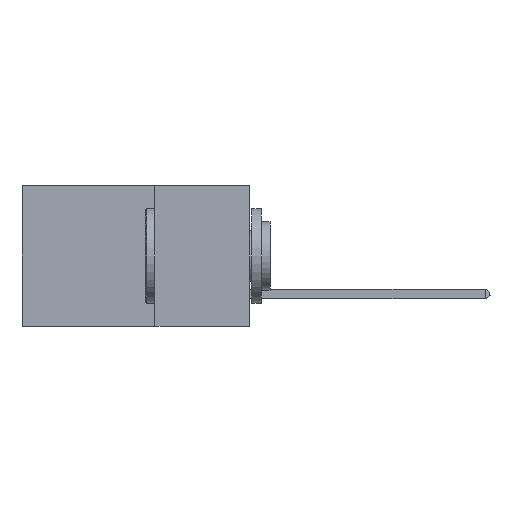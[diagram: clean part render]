
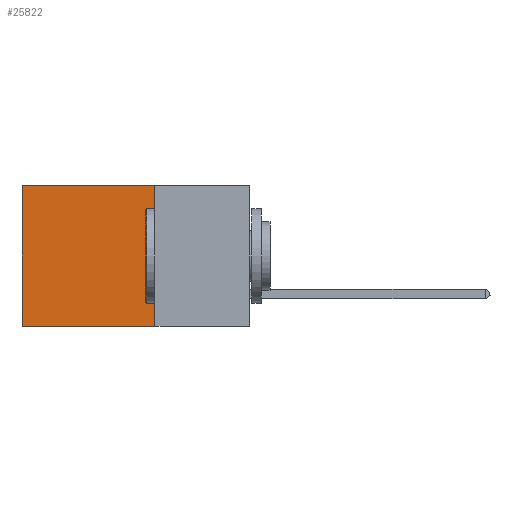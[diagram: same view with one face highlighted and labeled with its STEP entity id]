
A CAD part, left-side view. The second image highlights one B-rep face of the part: STEP entity #25822.
In plain terms, the highlighted planar face has unit normal (-1, 0, 0).
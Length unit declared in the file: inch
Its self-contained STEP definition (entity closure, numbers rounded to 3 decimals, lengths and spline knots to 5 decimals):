
#1035 = ORIENTED_EDGE ( 'NONE', *, *, #13545, .T. ) ;
#1721 = LINE ( 'NONE', #9431, #6981 ) ;
#2268 = ORIENTED_EDGE ( 'NONE', *, *, #10906, .T. ) ;
#4077 = DIRECTION ( 'NONE',  ( 0., 0., -1. ) ) ;
#4103 = VECTOR ( 'NONE', #25161, 39.37008 ) ;
#5337 = CARTESIAN_POINT ( 'NONE',  ( 0.2875, 0.6, 0. ) ) ;
#6981 = VECTOR ( 'NONE', #11683, 39.37008 ) ;
#7983 = VERTEX_POINT ( 'NONE', #5337 ) ;
#8752 = AXIS2_PLACEMENT_3D ( 'NONE', #27367, #15948, #20723 ) ;
#9068 = CARTESIAN_POINT ( 'NONE',  ( 0.2875, 0.25, 0. ) ) ;
#9376 = LINE ( 'NONE', #26934, #16824 ) ;
#9431 = CARTESIAN_POINT ( 'NONE',  ( 0.2875, 0.25, 0. ) ) ;
#10137 = LINE ( 'NONE', #22988, #4103 ) ;
#10906 = EDGE_CURVE ( 'NONE', #29170, #7983, #16612, .T. ) ;
#11400 = CARTESIAN_POINT ( 'NONE',  ( 0.2875, 0.25, -0.37 ) ) ;
#11448 = ORIENTED_EDGE ( 'NONE', *, *, #25806, .F. ) ;
#11585 = ORIENTED_EDGE ( 'NONE', *, *, #27945, .F. ) ;
#11683 = DIRECTION ( 'NONE',  ( 0., 0., -1. ) ) ;
#13518 = EDGE_LOOP ( 'NONE', ( #1035, #11585, #11448, #2268 ) ) ;
#13545 = EDGE_CURVE ( 'NONE', #7983, #23250, #9376, .T. ) ;
#13915 = CARTESIAN_POINT ( 'NONE',  ( 0.2875, 0.6, -0.37 ) ) ;
#15948 = DIRECTION ( 'NONE',  ( 1., 0., 0. ) ) ;
#16612 = LINE ( 'NONE', #9068, #28609 ) ;
#16824 = VECTOR ( 'NONE', #4077, 39.37008 ) ;
#20723 = DIRECTION ( 'NONE',  ( 0., 0., -1. ) ) ;
#21011 = VERTEX_POINT ( 'NONE', #11400 ) ;
#22988 = CARTESIAN_POINT ( 'NONE',  ( 0.2875, 0.25, -0.37 ) ) ;
#23250 = VERTEX_POINT ( 'NONE', #13915 ) ;
#24744 = CARTESIAN_POINT ( 'NONE',  ( 0.2875, 0.25, 0. ) ) ;
#25161 = DIRECTION ( 'NONE',  ( 0., 1., 0. ) ) ;
#25806 = EDGE_CURVE ( 'NONE', #29170, #21011, #1721, .T. ) ;
#25822 = ADVANCED_FACE ( 'NONE', ( #27819 ), #27461, .F. ) ;
#26934 = CARTESIAN_POINT ( 'NONE',  ( 0.2875, 0.6, 0. ) ) ;
#27101 = DIRECTION ( 'NONE',  ( 0., 1., 0. ) ) ;
#27367 = CARTESIAN_POINT ( 'NONE',  ( 0.2875, 0.25, 0. ) ) ;
#27461 = PLANE ( 'NONE',  #8752 ) ;
#27819 = FACE_OUTER_BOUND ( 'NONE', #13518, .T. ) ;
#27945 = EDGE_CURVE ( 'NONE', #21011, #23250, #10137, .T. ) ;
#28609 = VECTOR ( 'NONE', #27101, 39.37008 ) ;
#29170 = VERTEX_POINT ( 'NONE', #24744 ) ;
